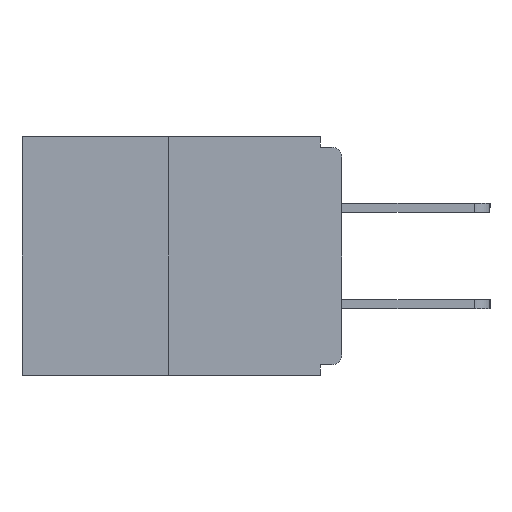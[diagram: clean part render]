
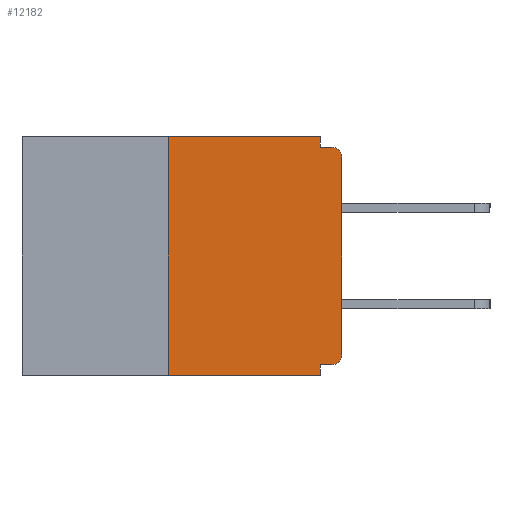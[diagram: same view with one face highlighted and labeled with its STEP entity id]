
A CAD part, left-side view. The second image highlights one B-rep face of the part: STEP entity #12182.
In plain terms, the highlighted planar face has unit normal (-1, 0, 0).
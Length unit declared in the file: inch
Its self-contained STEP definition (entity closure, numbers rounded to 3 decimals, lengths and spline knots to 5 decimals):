
#26 = VERTEX_POINT ( 'NONE', #2300 ) ;
#29 = LINE ( 'NONE', #8858, #9748 ) ;
#679 = EDGE_CURVE ( 'NONE', #15854, #20391, #1073, .T. ) ;
#1073 = LINE ( 'NONE', #18897, #17694 ) ;
#1191 = DIRECTION ( 'NONE',  ( 0., 0., 1. ) ) ;
#1609 = EDGE_CURVE ( 'NONE', #9406, #17051, #29, .T. ) ;
#2300 = CARTESIAN_POINT ( 'NONE',  ( 0., 0.25, 0. ) ) ;
#2530 = DIRECTION ( 'NONE',  ( -1., 0., 0. ) ) ;
#2553 = ORIENTED_EDGE ( 'NONE', *, *, #18254, .T. ) ;
#3119 = CARTESIAN_POINT ( 'NONE',  ( 0., 0.46, 0. ) ) ;
#3443 = LINE ( 'NONE', #13688, #16871 ) ;
#3688 = EDGE_CURVE ( 'NONE', #26, #21029, #7989, .T. ) ;
#3700 = CIRCLE ( 'NONE', #18378, 0.015 ) ;
#4172 = LINE ( 'NONE', #13142, #21528 ) ;
#4770 = ORIENTED_EDGE ( 'NONE', *, *, #679, .T. ) ;
#4930 = CARTESIAN_POINT ( 'NONE',  ( 0., 0.031, -0.328 ) ) ;
#4933 = CARTESIAN_POINT ( 'NONE',  ( 0., 0.015, -0.015 ) ) ;
#5614 = LINE ( 'NONE', #9144, #5846 ) ;
#5846 = VECTOR ( 'NONE', #12613, 39.37008 ) ;
#6187 = EDGE_LOOP ( 'NONE', ( #17325, #12855, #13700, #13018, #13510, #2553, #4770, #21296, #21105, #19591 ) ) ;
#6748 = EDGE_CURVE ( 'NONE', #20391, #19537, #17307, .T. ) ;
#7357 = CARTESIAN_POINT ( 'NONE',  ( 0., 0.25, -0.343 ) ) ;
#7540 = LINE ( 'NONE', #11096, #14708 ) ;
#7878 = CARTESIAN_POINT ( 'NONE',  ( 0., 0.46, 0. ) ) ;
#7976 = VERTEX_POINT ( 'NONE', #10472 ) ;
#7989 = LINE ( 'NONE', #7878, #21248 ) ;
#8702 = DIRECTION ( 'NONE',  ( 0., 0., -1. ) ) ;
#8858 = CARTESIAN_POINT ( 'NONE',  ( 0., 0., -0.328 ) ) ;
#9144 = CARTESIAN_POINT ( 'NONE',  ( 0., 0.46, -0.343 ) ) ;
#9406 = VERTEX_POINT ( 'NONE', #17953 ) ;
#9748 = VECTOR ( 'NONE', #15764, 39.37008 ) ;
#10119 = DIRECTION ( 'NONE',  ( 1., 0., 0. ) ) ;
#10472 = CARTESIAN_POINT ( 'NONE',  ( 0., 0.031, -0.015 ) ) ;
#10540 = DIRECTION ( 'NONE',  ( -1., 0., 0. ) ) ;
#11096 = CARTESIAN_POINT ( 'NONE',  ( 0., 0., -0.015 ) ) ;
#11461 = EDGE_CURVE ( 'NONE', #22214, #15216, #5614, .T. ) ;
#11477 = CARTESIAN_POINT ( 'NONE',  ( 0., 0.031, -0.343 ) ) ;
#11786 = DIRECTION ( 'NONE',  ( 0., 0., -1. ) ) ;
#11866 = PLANE ( 'NONE',  #12860 ) ;
#11938 = EDGE_CURVE ( 'NONE', #21029, #7976, #4172, .T. ) ;
#12044 = CARTESIAN_POINT ( 'NONE',  ( 0., 0., -0.313 ) ) ;
#12182 = ADVANCED_FACE ( 'NONE', ( #22570 ), #11866, .F. ) ;
#12584 = AXIS2_PLACEMENT_3D ( 'NONE', #15723, #10540, #8702 ) ;
#12613 = DIRECTION ( 'NONE',  ( 0., -1., 0. ) ) ;
#12634 = EDGE_CURVE ( 'NONE', #7976, #19537, #7540, .T. ) ;
#12727 = EDGE_CURVE ( 'NONE', #17051, #15216, #18230, .T. ) ;
#12855 = ORIENTED_EDGE ( 'NONE', *, *, #15435, .F. ) ;
#12860 = AXIS2_PLACEMENT_3D ( 'NONE', #3119, #10119, #17144 ) ;
#13018 = ORIENTED_EDGE ( 'NONE', *, *, #12727, .F. ) ;
#13142 = CARTESIAN_POINT ( 'NONE',  ( 0., 0.031, 0. ) ) ;
#13510 = ORIENTED_EDGE ( 'NONE', *, *, #1609, .F. ) ;
#13688 = CARTESIAN_POINT ( 'NONE',  ( 0., 0.25, 0. ) ) ;
#13700 = ORIENTED_EDGE ( 'NONE', *, *, #11461, .T. ) ;
#14708 = VECTOR ( 'NONE', #21594, 39.37008 ) ;
#14727 = CARTESIAN_POINT ( 'NONE',  ( 0., 0.015, -0.313 ) ) ;
#15216 = VERTEX_POINT ( 'NONE', #11477 ) ;
#15435 = EDGE_CURVE ( 'NONE', #22214, #26, #3443, .T. ) ;
#15723 = CARTESIAN_POINT ( 'NONE',  ( 0., 0.015, -0.03 ) ) ;
#15741 = DIRECTION ( 'NONE',  ( 0., 0., 1. ) ) ;
#15764 = DIRECTION ( 'NONE',  ( 0., 1., 0. ) ) ;
#15854 = VERTEX_POINT ( 'NONE', #12044 ) ;
#16333 = DIRECTION ( 'NONE',  ( 0., 0., -1. ) ) ;
#16871 = VECTOR ( 'NONE', #15741, 39.37008 ) ;
#17051 = VERTEX_POINT ( 'NONE', #4930 ) ;
#17064 = CARTESIAN_POINT ( 'NONE',  ( 0., 0.031, -0.343 ) ) ;
#17144 = DIRECTION ( 'NONE',  ( 0., 0., -1. ) ) ;
#17307 = CIRCLE ( 'NONE', #12584, 0.015 ) ;
#17325 = ORIENTED_EDGE ( 'NONE', *, *, #3688, .F. ) ;
#17639 = VECTOR ( 'NONE', #11786, 39.37008 ) ;
#17694 = VECTOR ( 'NONE', #1191, 39.37008 ) ;
#17953 = CARTESIAN_POINT ( 'NONE',  ( 0., 0.015, -0.328 ) ) ;
#18230 = LINE ( 'NONE', #17064, #17639 ) ;
#18254 = EDGE_CURVE ( 'NONE', #9406, #15854, #3700, .T. ) ;
#18378 = AXIS2_PLACEMENT_3D ( 'NONE', #14727, #2530, #16333 ) ;
#18897 = CARTESIAN_POINT ( 'NONE',  ( 0., 0., 0. ) ) ;
#19001 = CARTESIAN_POINT ( 'NONE',  ( 0., 0., -0.03 ) ) ;
#19537 = VERTEX_POINT ( 'NONE', #4933 ) ;
#19591 = ORIENTED_EDGE ( 'NONE', *, *, #11938, .F. ) ;
#20158 = DIRECTION ( 'NONE',  ( 0., 0., -1. ) ) ;
#20323 = CARTESIAN_POINT ( 'NONE',  ( 0., 0.031, 0. ) ) ;
#20391 = VERTEX_POINT ( 'NONE', #19001 ) ;
#21029 = VERTEX_POINT ( 'NONE', #20323 ) ;
#21105 = ORIENTED_EDGE ( 'NONE', *, *, #12634, .F. ) ;
#21248 = VECTOR ( 'NONE', #21928, 39.37008 ) ;
#21296 = ORIENTED_EDGE ( 'NONE', *, *, #6748, .T. ) ;
#21528 = VECTOR ( 'NONE', #20158, 39.37008 ) ;
#21594 = DIRECTION ( 'NONE',  ( 0., -1., 0. ) ) ;
#21928 = DIRECTION ( 'NONE',  ( 0., -1., 0. ) ) ;
#22214 = VERTEX_POINT ( 'NONE', #7357 ) ;
#22570 = FACE_OUTER_BOUND ( 'NONE', #6187, .T. ) ;
